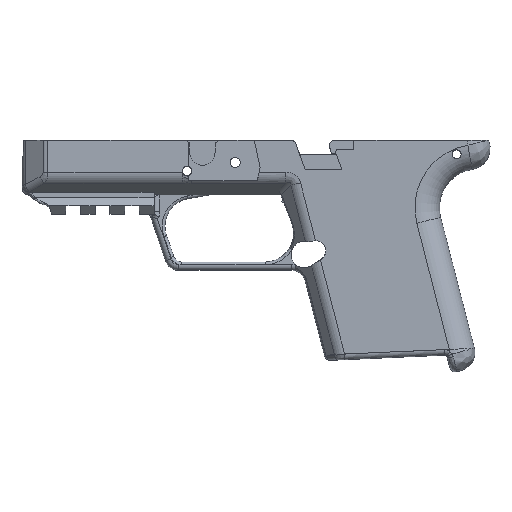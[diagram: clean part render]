
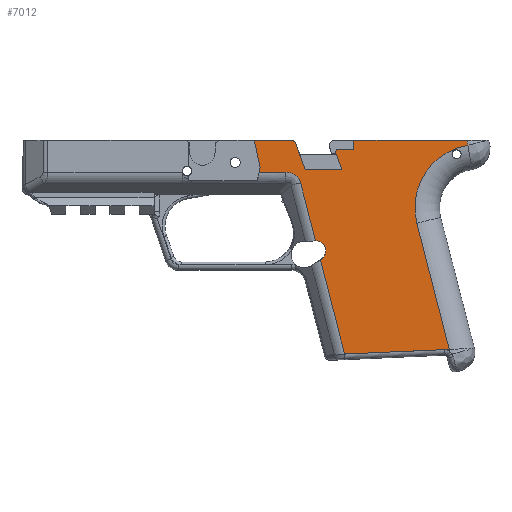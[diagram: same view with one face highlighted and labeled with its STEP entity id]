
A CAD part, left-side view. The second image highlights one B-rep face of the part: STEP entity #7012.
In plain terms, the highlighted face is planar.
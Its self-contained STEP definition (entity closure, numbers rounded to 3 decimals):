
#122=PLANE('',#7465);
#466=ELLIPSE('',#7467,10.693,7.);
#647=FACE_OUTER_BOUND('',#1040,.T.);
#1040=EDGE_LOOP('',(#5015,#5016,#5017,#5018,#5019,#5020,#5021,#5022,#5023,
#5024,#5025,#5026,#5027,#5028,#5029,#5030,#5031,#5032,#5033,#5034,#5035,
#5036,#5037));
#1519=LINE('',#11164,#2153);
#1520=LINE('',#11166,#2154);
#1521=LINE('',#11168,#2155);
#1522=LINE('',#11172,#2156);
#1523=LINE('',#11174,#2157);
#1524=LINE('',#11176,#2158);
#1525=LINE('',#11178,#2159);
#1526=LINE('',#11182,#2160);
#1527=LINE('',#11190,#2161);
#1528=LINE('',#11192,#2162);
#1529=LINE('',#11194,#2163);
#1530=LINE('',#11196,#2164);
#1531=LINE('',#11202,#2165);
#1532=LINE('',#11204,#2166);
#1533=LINE('',#11205,#2167);
#2153=VECTOR('',#8400,10.);
#2154=VECTOR('',#8401,10.);
#2155=VECTOR('',#8402,10.);
#2156=VECTOR('',#8405,10.);
#2157=VECTOR('',#8406,10.);
#2158=VECTOR('',#8407,10.);
#2159=VECTOR('',#8408,10.);
#2160=VECTOR('',#8411,10.);
#2161=VECTOR('',#8418,10.);
#2162=VECTOR('',#8419,10.);
#2163=VECTOR('',#8420,10.);
#2164=VECTOR('',#8421,10.);
#2165=VECTOR('',#8426,10.);
#2166=VECTOR('',#8427,10.);
#2167=VECTOR('',#8428,10.);
#2674=CIRCLE('',#7464,1.);
#2675=CIRCLE('',#7466,2.);
#2676=CIRCLE('',#7468,3.585);
#2677=CIRCLE('',#7469,2.921);
#2678=CIRCLE('',#7470,3.585);
#2679=CIRCLE('',#7471,22.475);
#2680=CIRCLE('',#7472,7.5);
#3007=VERTEX_POINT('',#11157);
#3008=VERTEX_POINT('',#11159);
#3009=VERTEX_POINT('',#11163);
#3010=VERTEX_POINT('',#11165);
#3011=VERTEX_POINT('',#11167);
#3012=VERTEX_POINT('',#11169);
#3013=VERTEX_POINT('',#11171);
#3014=VERTEX_POINT('',#11173);
#3015=VERTEX_POINT('',#11175);
#3016=VERTEX_POINT('',#11177);
#3017=VERTEX_POINT('',#11179);
#3018=VERTEX_POINT('',#11181);
#3019=VERTEX_POINT('',#11183);
#3020=VERTEX_POINT('',#11185);
#3021=VERTEX_POINT('',#11187);
#3022=VERTEX_POINT('',#11189);
#3023=VERTEX_POINT('',#11191);
#3024=VERTEX_POINT('',#11193);
#3025=VERTEX_POINT('',#11195);
#3026=VERTEX_POINT('',#11197);
#3027=VERTEX_POINT('',#11199);
#3028=VERTEX_POINT('',#11201);
#3029=VERTEX_POINT('',#11203);
#3766=EDGE_CURVE('',#3007,#3008,#2674,.T.);
#3768=EDGE_CURVE('',#3007,#3009,#1519,.F.);
#3769=EDGE_CURVE('',#3009,#3010,#1520,.T.);
#3770=EDGE_CURVE('',#3010,#3011,#1521,.F.);
#3771=EDGE_CURVE('',#3012,#3011,#2675,.T.);
#3772=EDGE_CURVE('',#3012,#3013,#1522,.T.);
#3773=EDGE_CURVE('',#3013,#3014,#1523,.T.);
#3774=EDGE_CURVE('',#3014,#3015,#1524,.T.);
#3775=EDGE_CURVE('',#3016,#3015,#1525,.T.);
#3776=EDGE_CURVE('',#3017,#3016,#466,.T.);
#3777=EDGE_CURVE('',#3018,#3017,#1526,.T.);
#3778=EDGE_CURVE('',#3018,#3019,#2676,.T.);
#3779=EDGE_CURVE('',#3019,#3020,#2677,.T.);
#3780=EDGE_CURVE('',#3020,#3021,#2678,.T.);
#3781=EDGE_CURVE('',#3021,#3022,#1527,.T.);
#3782=EDGE_CURVE('',#3023,#3022,#1528,.T.);
#3783=EDGE_CURVE('',#3024,#3023,#1529,.T.);
#3784=EDGE_CURVE('',#3025,#3024,#1530,.T.);
#3785=EDGE_CURVE('',#3026,#3025,#2679,.T.);
#3786=EDGE_CURVE('',#3027,#3026,#2680,.T.);
#3787=EDGE_CURVE('',#3027,#3028,#1531,.T.);
#3788=EDGE_CURVE('',#3028,#3029,#1532,.F.);
#3789=EDGE_CURVE('',#3029,#3008,#1533,.T.);
#5015=ORIENTED_EDGE('',*,*,#3766,.F.);
#5016=ORIENTED_EDGE('',*,*,#3768,.T.);
#5017=ORIENTED_EDGE('',*,*,#3769,.T.);
#5018=ORIENTED_EDGE('',*,*,#3770,.T.);
#5019=ORIENTED_EDGE('',*,*,#3771,.F.);
#5020=ORIENTED_EDGE('',*,*,#3772,.T.);
#5021=ORIENTED_EDGE('',*,*,#3773,.T.);
#5022=ORIENTED_EDGE('',*,*,#3774,.T.);
#5023=ORIENTED_EDGE('',*,*,#3775,.F.);
#5024=ORIENTED_EDGE('',*,*,#3776,.F.);
#5025=ORIENTED_EDGE('',*,*,#3777,.F.);
#5026=ORIENTED_EDGE('',*,*,#3778,.T.);
#5027=ORIENTED_EDGE('',*,*,#3779,.T.);
#5028=ORIENTED_EDGE('',*,*,#3780,.T.);
#5029=ORIENTED_EDGE('',*,*,#3781,.T.);
#5030=ORIENTED_EDGE('',*,*,#3782,.F.);
#5031=ORIENTED_EDGE('',*,*,#3783,.F.);
#5032=ORIENTED_EDGE('',*,*,#3784,.F.);
#5033=ORIENTED_EDGE('',*,*,#3785,.F.);
#5034=ORIENTED_EDGE('',*,*,#3786,.F.);
#5035=ORIENTED_EDGE('',*,*,#3787,.T.);
#5036=ORIENTED_EDGE('',*,*,#3788,.T.);
#5037=ORIENTED_EDGE('',*,*,#3789,.T.);
#7012=ADVANCED_FACE('',(#647),#122,.F.);
#7464=AXIS2_PLACEMENT_3D('',#11160,#8395,#8396);
#7465=AXIS2_PLACEMENT_3D('',#11162,#8398,#8399);
#7466=AXIS2_PLACEMENT_3D('',#11170,#8403,#8404);
#7467=AXIS2_PLACEMENT_3D('',#11180,#8409,#8410);
#7468=AXIS2_PLACEMENT_3D('',#11184,#8412,#8413);
#7469=AXIS2_PLACEMENT_3D('',#11186,#8414,#8415);
#7470=AXIS2_PLACEMENT_3D('',#11188,#8416,#8417);
#7471=AXIS2_PLACEMENT_3D('',#11198,#8422,#8423);
#7472=AXIS2_PLACEMENT_3D('',#11200,#8424,#8425);
#8395=DIRECTION('center_axis',(-1.,0.,0.));
#8396=DIRECTION('ref_axis',(0.,0.817,-0.576));
#8398=DIRECTION('center_axis',(-1.,0.,0.));
#8399=DIRECTION('ref_axis',(0.,1.,0.));
#8400=DIRECTION('',(0.,0.336,-0.942));
#8401=DIRECTION('',(0.,1.,0.));
#8402=DIRECTION('',(0.,-0.336,0.942));
#8403=DIRECTION('center_axis',(-1.,0.,0.));
#8404=DIRECTION('ref_axis',(0.,-0.576,-0.817));
#8405=DIRECTION('',(0.,1.,0.));
#8406=DIRECTION('',(0.,-0.21,0.978));
#8407=DIRECTION('',(0.,0.21,0.978));
#8408=DIRECTION('',(0.,1.,0.));
#8409=DIRECTION('center_axis',(1.,0.,0.));
#8410=DIRECTION('ref_axis',(0.,-0.714,-0.7));
#8411=DIRECTION('',(0.,0.249,-0.969));
#8412=DIRECTION('center_axis',(-1.,0.,0.));
#8413=DIRECTION('ref_axis',(0.,1.,0.));
#8414=DIRECTION('center_axis',(-1.,0.,0.));
#8415=DIRECTION('ref_axis',(0.,1.,0.));
#8416=DIRECTION('center_axis',(-1.,0.,0.));
#8417=DIRECTION('ref_axis',(0.,1.,0.));
#8418=DIRECTION('',(0.,0.828,0.56));
#8419=DIRECTION('',(0.,0.249,-0.969));
#8420=DIRECTION('',(0.,0.999,0.044));
#8421=DIRECTION('',(0.,-0.249,0.969));
#8422=DIRECTION('center_axis',(1.,0.,0.));
#8423=DIRECTION('ref_axis',(0.,0.,
1.));
#8424=DIRECTION('center_axis',(1.,0.,0.));
#8425=DIRECTION('ref_axis',(0.,-0.97,-0.244));
#8426=DIRECTION('',(0.,1.,0.));
#8427=DIRECTION('',(0.,0.,-1.));
#8428=DIRECTION('',(0.,1.,0.));
#11157=CARTESIAN_POINT('',(22.175,-32.374,-2.995));
#11159=CARTESIAN_POINT('',(22.175,-33.316,-4.331));
#11160=CARTESIAN_POINT('Origin',(22.175,-33.316,-3.331));
#11162=CARTESIAN_POINT('Origin',(22.175,-5.921,2.186));
#11163=CARTESIAN_POINT('',(22.175,-34.514,3.));
#11164=CARTESIAN_POINT('',(22.175,-30.976,-6.913));
#11165=CARTESIAN_POINT('',(22.175,-21.407,3.));
#11166=CARTESIAN_POINT('',(22.175,-21.764,3.));
#11167=CARTESIAN_POINT('',(22.175,-18.114,-6.228));
#11168=CARTESIAN_POINT('',(22.175,-19.552,-2.199));
#11169=CARTESIAN_POINT('',(22.175,-16.23,-7.556));
#11170=CARTESIAN_POINT('Origin',(22.175,-16.23,-5.556));
#11171=CARTESIAN_POINT('',(22.175,-3.3,-7.556));
#11172=CARTESIAN_POINT('',(22.175,-84.951,-7.556));
#11173=CARTESIAN_POINT('',(22.175,-5.389,2.186));
#11174=CARTESIAN_POINT('',(22.175,-4.356,-2.63));
#11175=CARTESIAN_POINT('',(22.175,-5.025,3.884));
#11176=CARTESIAN_POINT('',(22.175,-5.4,2.132));
#11177=CARTESIAN_POINT('',(22.175,-14.536,3.884));
#11178=CARTESIAN_POINT('',(22.175,35.814,3.884));
#11179=CARTESIAN_POINT('',(22.175,-19.783,7.651));
#11180=CARTESIAN_POINT('Origin',(22.175,-10.907,12.884));
#11181=CARTESIAN_POINT('',(22.175,-25.074,28.233));
#11182=CARTESIAN_POINT('',(22.175,-24.659,26.619));
#11183=CARTESIAN_POINT('',(22.175,-28.502,30.561));
#11184=CARTESIAN_POINT('Origin',(22.175,-25.144,31.817));
#11185=CARTESIAN_POINT('',(22.175,-28.617,30.925));
#11186=CARTESIAN_POINT('Origin',(22.175,-25.779,31.618));
#11187=CARTESIAN_POINT('',(22.175,-27.153,34.787));
#11188=CARTESIAN_POINT('Origin',(22.175,-25.144,31.817));
#11189=CARTESIAN_POINT('',(22.175,-26.817,35.014));
#11190=CARTESIAN_POINT('',(22.175,-25.054,36.207));
#11191=CARTESIAN_POINT('',(22.175,-35.447,68.587));
#11192=CARTESIAN_POINT('',(22.175,-24.659,26.619));
#11193=CARTESIAN_POINT('',(22.175,-72.722,66.935));
#11194=CARTESIAN_POINT('',(22.175,-38.785,68.439));
#11195=CARTESIAN_POINT('',(22.175,-61.184,22.049));
#11196=CARTESIAN_POINT('',(22.175,-73.103,68.418));
#11197=CARTESIAN_POINT('',(22.175,-79.332,-5.728));
#11198=CARTESIAN_POINT('Origin',(22.175,-82.951,16.453));
#11199=CARTESIAN_POINT('',(22.175,-79.106,-7.556));
#11200=CARTESIAN_POINT('Origin',(22.175,-86.606,-7.556));
#11201=CARTESIAN_POINT('',(22.175,-38.774,-7.556));
#11202=CARTESIAN_POINT('',(22.175,-82.951,-7.556));
#11203=CARTESIAN_POINT('',(22.175,-38.774,-4.331));
#11204=CARTESIAN_POINT('',(22.175,-38.774,-2.685));
#11205=CARTESIAN_POINT('',(22.175,-18.598,-4.331));
